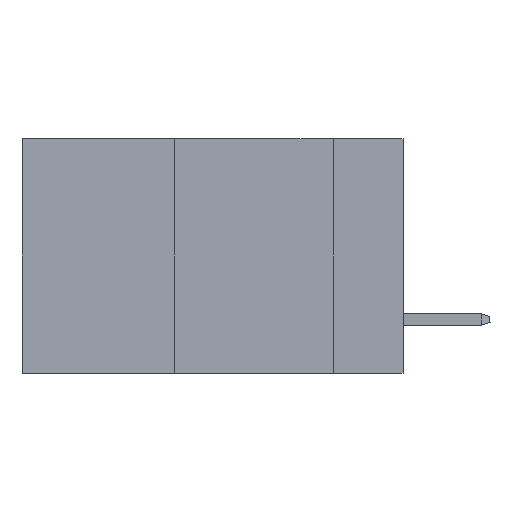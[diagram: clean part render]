
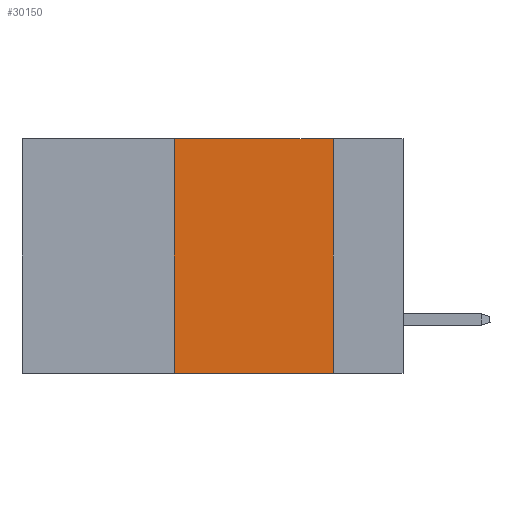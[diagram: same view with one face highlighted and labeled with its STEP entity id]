
A CAD part, left-side view. The second image highlights one B-rep face of the part: STEP entity #30150.
In plain terms, the highlighted planar face has unit normal (-1, 0, 0).
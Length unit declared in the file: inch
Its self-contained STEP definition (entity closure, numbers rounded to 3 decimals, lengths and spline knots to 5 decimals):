
#1165 = LINE ( 'NONE', #1729, #22052 ) ;
#1374 = EDGE_CURVE ( 'NONE', #7627, #23830, #1165, .T. ) ;
#1729 = CARTESIAN_POINT ( 'NONE',  ( 0., 0.6, -0.37 ) ) ;
#2137 = EDGE_LOOP ( 'NONE', ( #4851, #26136, #33994, #2377 ) ) ;
#2377 = ORIENTED_EDGE ( 'NONE', *, *, #1374, .T. ) ;
#3740 = FACE_OUTER_BOUND ( 'NONE', #2137, .T. ) ;
#4851 = ORIENTED_EDGE ( 'NONE', *, *, #9476, .F. ) ;
#4857 = VERTEX_POINT ( 'NONE', #31278 ) ;
#6378 = PLANE ( 'NONE',  #33647 ) ;
#7452 = LINE ( 'NONE', #12848, #34283 ) ;
#7627 = VERTEX_POINT ( 'NONE', #33258 ) ;
#9476 = EDGE_CURVE ( 'NONE', #4857, #23830, #26812, .T. ) ;
#12136 = CARTESIAN_POINT ( 'NONE',  ( 0., 0.11, 0. ) ) ;
#12848 = CARTESIAN_POINT ( 'NONE',  ( 0., 0.36, 0. ) ) ;
#13087 = DIRECTION ( 'NONE',  ( 0., -1., 0. ) ) ;
#13991 = LINE ( 'NONE', #16602, #22832 ) ;
#16602 = CARTESIAN_POINT ( 'NONE',  ( 0., 0.6, 0. ) ) ;
#17740 = DIRECTION ( 'NONE',  ( 0., 0., -1. ) ) ;
#19149 = EDGE_CURVE ( 'NONE', #7627, #32857, #7452, .T. ) ;
#20495 = DIRECTION ( 'NONE',  ( 0., 0., -1. ) ) ;
#22052 = VECTOR ( 'NONE', #13087, 39.37008 ) ;
#22832 = VECTOR ( 'NONE', #25694, 39.37008 ) ;
#23830 = VERTEX_POINT ( 'NONE', #26917 ) ;
#25694 = DIRECTION ( 'NONE',  ( 0., -1., 0. ) ) ;
#26136 = ORIENTED_EDGE ( 'NONE', *, *, #31122, .F. ) ;
#26265 = DIRECTION ( 'NONE',  ( 1., 0., 0. ) ) ;
#26812 = LINE ( 'NONE', #12136, #26822 ) ;
#26822 = VECTOR ( 'NONE', #20495, 39.37008 ) ;
#26917 = CARTESIAN_POINT ( 'NONE',  ( 0., 0.11, -0.37 ) ) ;
#30150 = ADVANCED_FACE ( 'NONE', ( #3740 ), #6378, .F. ) ;
#30298 = DIRECTION ( 'NONE',  ( 0., 0., 1. ) ) ;
#31122 = EDGE_CURVE ( 'NONE', #32857, #4857, #13991, .T. ) ;
#31278 = CARTESIAN_POINT ( 'NONE',  ( 0., 0.11, 0. ) ) ;
#32857 = VERTEX_POINT ( 'NONE', #34018 ) ;
#33258 = CARTESIAN_POINT ( 'NONE',  ( 0., 0.36, -0.37 ) ) ;
#33647 = AXIS2_PLACEMENT_3D ( 'NONE', #35601, #26265, #17740 ) ;
#33994 = ORIENTED_EDGE ( 'NONE', *, *, #19149, .F. ) ;
#34018 = CARTESIAN_POINT ( 'NONE',  ( 0., 0.36, 0. ) ) ;
#34283 = VECTOR ( 'NONE', #30298, 39.37008 ) ;
#35601 = CARTESIAN_POINT ( 'NONE',  ( 0., 0.6, 0. ) ) ;
